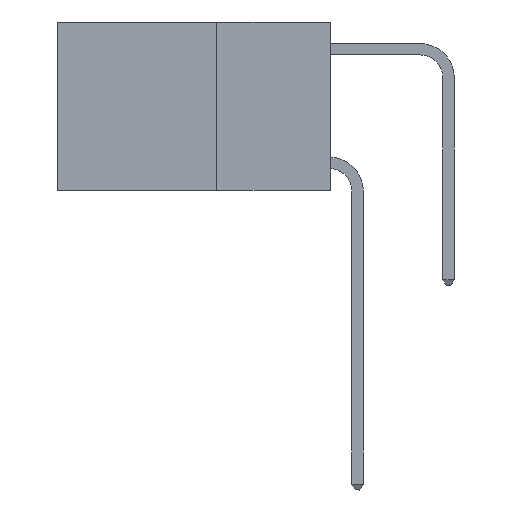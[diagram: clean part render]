
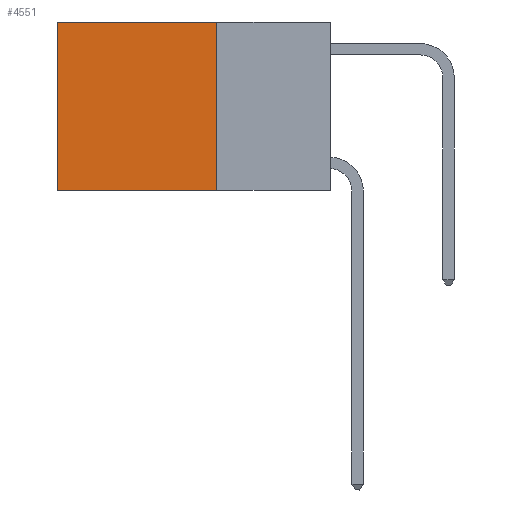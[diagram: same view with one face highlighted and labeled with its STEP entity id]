
A CAD part, left-side view. The second image highlights one B-rep face of the part: STEP entity #4551.
In plain terms, the highlighted planar face has unit normal (-1, 0, 0).
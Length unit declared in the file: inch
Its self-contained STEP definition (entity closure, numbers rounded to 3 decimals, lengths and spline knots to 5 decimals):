
#92 = DIRECTION ( 'NONE',  ( 0., 1., 0. ) ) ;
#234 = LINE ( 'NONE', #11000, #10830 ) ;
#2508 = VECTOR ( 'NONE', #8259, 39.37008 ) ;
#2674 = DIRECTION ( 'NONE',  ( 1., 0., 0. ) ) ;
#2820 = LINE ( 'NONE', #3487, #2508 ) ;
#3487 = CARTESIAN_POINT ( 'NONE',  ( 0.2625, 0.25, 0. ) ) ;
#3791 = CARTESIAN_POINT ( 'NONE',  ( 0.2625, 0.25, -0.37 ) ) ;
#4220 = CARTESIAN_POINT ( 'NONE',  ( 0.2625, 0.6, 0. ) ) ;
#4551 = ADVANCED_FACE ( 'NONE', ( #11677 ), #10834, .F. ) ;
#4766 = ORIENTED_EDGE ( 'NONE', *, *, #9219, .F. ) ;
#4863 = EDGE_LOOP ( 'NONE', ( #10416, #7679, #4766, #7720 ) ) ;
#5618 = EDGE_CURVE ( 'NONE', #9521, #11945, #234, .T. ) ;
#5645 = VERTEX_POINT ( 'NONE', #4220 ) ;
#6083 = CARTESIAN_POINT ( 'NONE',  ( 0.2625, 0.25, 0. ) ) ;
#6398 = LINE ( 'NONE', #11970, #7678 ) ;
#6628 = LINE ( 'NONE', #8705, #11075 ) ;
#7678 = VECTOR ( 'NONE', #12996, 39.37008 ) ;
#7679 = ORIENTED_EDGE ( 'NONE', *, *, #5618, .F. ) ;
#7720 = ORIENTED_EDGE ( 'NONE', *, *, #9353, .T. ) ;
#7788 = DIRECTION ( 'NONE',  ( 0., 0., -1. ) ) ;
#8259 = DIRECTION ( 'NONE',  ( 0., 0., -1. ) ) ;
#8427 = AXIS2_PLACEMENT_3D ( 'NONE', #11782, #2674, #7788 ) ;
#8705 = CARTESIAN_POINT ( 'NONE',  ( 0.2625, 0.25, 0. ) ) ;
#9219 = EDGE_CURVE ( 'NONE', #11823, #9521, #2820, .T. ) ;
#9353 = EDGE_CURVE ( 'NONE', #11823, #5645, #6628, .T. ) ;
#9521 = VERTEX_POINT ( 'NONE', #3791 ) ;
#10416 = ORIENTED_EDGE ( 'NONE', *, *, #12063, .T. ) ;
#10830 = VECTOR ( 'NONE', #92, 39.37008 ) ;
#10834 = PLANE ( 'NONE',  #8427 ) ;
#11000 = CARTESIAN_POINT ( 'NONE',  ( 0.2625, 0.25, -0.37 ) ) ;
#11075 = VECTOR ( 'NONE', #11832, 39.37008 ) ;
#11391 = CARTESIAN_POINT ( 'NONE',  ( 0.2625, 0.6, -0.37 ) ) ;
#11677 = FACE_OUTER_BOUND ( 'NONE', #4863, .T. ) ;
#11782 = CARTESIAN_POINT ( 'NONE',  ( 0.2625, 0.25, 0. ) ) ;
#11823 = VERTEX_POINT ( 'NONE', #6083 ) ;
#11832 = DIRECTION ( 'NONE',  ( 0., 1., 0. ) ) ;
#11945 = VERTEX_POINT ( 'NONE', #11391 ) ;
#11970 = CARTESIAN_POINT ( 'NONE',  ( 0.2625, 0.6, 0. ) ) ;
#12063 = EDGE_CURVE ( 'NONE', #5645, #11945, #6398, .T. ) ;
#12996 = DIRECTION ( 'NONE',  ( 0., 0., -1. ) ) ;
